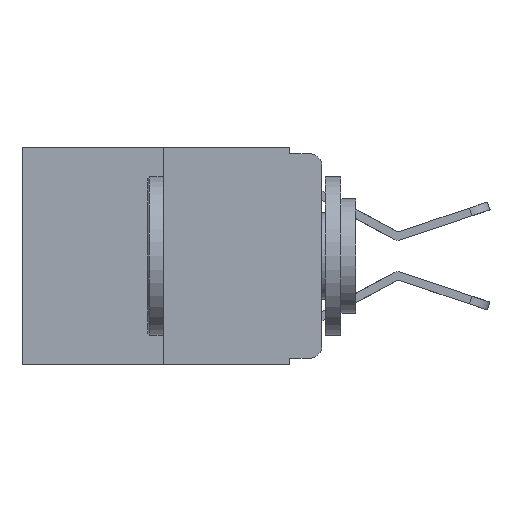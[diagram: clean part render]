
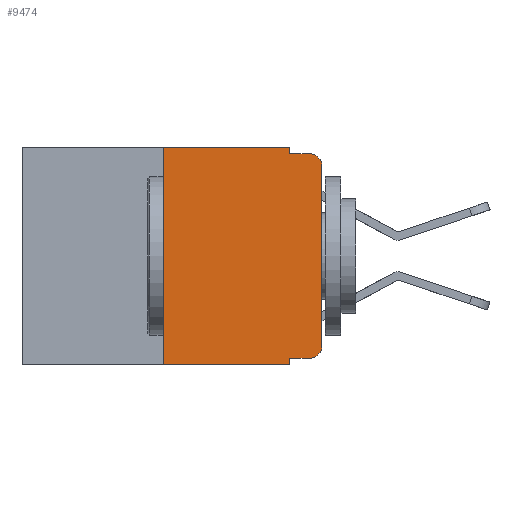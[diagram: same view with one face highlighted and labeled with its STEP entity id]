
A CAD part, left-side view. The second image highlights one B-rep face of the part: STEP entity #9474.
In plain terms, the highlighted planar face has unit normal (-1, 0, 0).
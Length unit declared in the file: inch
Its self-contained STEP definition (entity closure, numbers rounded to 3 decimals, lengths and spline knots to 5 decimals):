
#165 = DIRECTION ( 'NONE',  ( -1., 0., 0. ) ) ;
#377 = EDGE_CURVE ( 'NONE', #1621, #12043, #16840, .T. ) ;
#476 = CARTESIAN_POINT ( 'NONE',  ( 0., 0.051, -0.333 ) ) ;
#482 = CARTESIAN_POINT ( 'NONE',  ( 0., 0.051, -0.343 ) ) ;
#500 = VERTEX_POINT ( 'NONE', #15904 ) ;
#511 = EDGE_CURVE ( 'NONE', #15397, #2611, #18516, .T. ) ;
#589 = DIRECTION ( 'NONE',  ( 0., -1., 0. ) ) ;
#1621 = VERTEX_POINT ( 'NONE', #9645 ) ;
#1849 = PLANE ( 'NONE',  #20165 ) ;
#2248 = CIRCLE ( 'NONE', #12895, 0.02 ) ;
#2607 = CARTESIAN_POINT ( 'NONE',  ( 0., 0.473, -0.343 ) ) ;
#2611 = VERTEX_POINT ( 'NONE', #8493 ) ;
#2838 = ORIENTED_EDGE ( 'NONE', *, *, #20368, .T. ) ;
#3014 = VECTOR ( 'NONE', #19386, 39.37008 ) ;
#3291 = DIRECTION ( 'NONE',  ( 0., -1., 0. ) ) ;
#3378 = ORIENTED_EDGE ( 'NONE', *, *, #19338, .F. ) ;
#3545 = DIRECTION ( 'NONE',  ( 1., 0., 0. ) ) ;
#3826 = CARTESIAN_POINT ( 'NONE',  ( 0., 0.25, -0.343 ) ) ;
#3952 = VERTEX_POINT ( 'NONE', #3826 ) ;
#4013 = VECTOR ( 'NONE', #20763, 39.37008 ) ;
#4062 = VECTOR ( 'NONE', #3291, 39.37008 ) ;
#4450 = VECTOR ( 'NONE', #13975, 39.37008 ) ;
#4675 = EDGE_CURVE ( 'NONE', #3952, #16261, #12667, .T. ) ;
#5252 = ORIENTED_EDGE ( 'NONE', *, *, #16253, .F. ) ;
#5303 = DIRECTION ( 'NONE',  ( -1., 0., 0. ) ) ;
#5996 = ORIENTED_EDGE ( 'NONE', *, *, #18322, .F. ) ;
#6237 = ORIENTED_EDGE ( 'NONE', *, *, #511, .T. ) ;
#6366 = CARTESIAN_POINT ( 'NONE',  ( 0., 0., 0. ) ) ;
#6499 = ORIENTED_EDGE ( 'NONE', *, *, #377, .F. ) ;
#6713 = VECTOR ( 'NONE', #10400, 39.37008 ) ;
#6900 = CIRCLE ( 'NONE', #15809, 0.02 ) ;
#7520 = CARTESIAN_POINT ( 'NONE',  ( 0., 0.051, -0.333 ) ) ;
#7838 = FACE_OUTER_BOUND ( 'NONE', #12931, .T. ) ;
#8493 = CARTESIAN_POINT ( 'NONE',  ( 0., 0., -0.03 ) ) ;
#8799 = CARTESIAN_POINT ( 'NONE',  ( 0., 0.051, 0. ) ) ;
#8902 = CARTESIAN_POINT ( 'NONE',  ( 0., 0.051, -0.01 ) ) ;
#9474 = ADVANCED_FACE ( 'NONE', ( #7838 ), #1849, .F. ) ;
#9645 = CARTESIAN_POINT ( 'NONE',  ( 0., 0.25, 0. ) ) ;
#10112 = CARTESIAN_POINT ( 'NONE',  ( 0., 0.02, -0.03 ) ) ;
#10400 = DIRECTION ( 'NONE',  ( 0., 0., -1. ) ) ;
#10975 = VECTOR ( 'NONE', #589, 39.37008 ) ;
#10991 = LINE ( 'NONE', #18878, #15260 ) ;
#11568 = DIRECTION ( 'NONE',  ( 0., 0., 1. ) ) ;
#11703 = DIRECTION ( 'NONE',  ( 0., 0., -1. ) ) ;
#12043 = VERTEX_POINT ( 'NONE', #14399 ) ;
#12667 = LINE ( 'NONE', #2607, #4062 ) ;
#12895 = AXIS2_PLACEMENT_3D ( 'NONE', #14918, #5303, #16499 ) ;
#12931 = EDGE_LOOP ( 'NONE', ( #6237, #2838, #3378, #5996, #6499, #19642, #20609, #5252, #14808, #16291 ) ) ;
#13274 = CARTESIAN_POINT ( 'NONE',  ( 0., 0.473, 0. ) ) ;
#13975 = DIRECTION ( 'NONE',  ( 0., -1., 0. ) ) ;
#14120 = EDGE_CURVE ( 'NONE', #500, #15397, #2248, .T. ) ;
#14399 = CARTESIAN_POINT ( 'NONE',  ( 0., 0.051, 0. ) ) ;
#14584 = VERTEX_POINT ( 'NONE', #16076 ) ;
#14808 = ORIENTED_EDGE ( 'NONE', *, *, #15193, .T. ) ;
#14865 = VECTOR ( 'NONE', #11568, 39.37008 ) ;
#14873 = DIRECTION ( 'NONE',  ( 0., 0., -1. ) ) ;
#14918 = CARTESIAN_POINT ( 'NONE',  ( 0., 0.02, -0.313 ) ) ;
#15193 = EDGE_CURVE ( 'NONE', #18071, #500, #17744, .T. ) ;
#15260 = VECTOR ( 'NONE', #15777, 39.37008 ) ;
#15397 = VERTEX_POINT ( 'NONE', #20687 ) ;
#15777 = DIRECTION ( 'NONE',  ( 0., 0., -1. ) ) ;
#15809 = AXIS2_PLACEMENT_3D ( 'NONE', #10112, #165, #11703 ) ;
#15904 = CARTESIAN_POINT ( 'NONE',  ( 0., 0.02, -0.333 ) ) ;
#16076 = CARTESIAN_POINT ( 'NONE',  ( 0., 0.02, -0.01 ) ) ;
#16253 = EDGE_CURVE ( 'NONE', #18071, #16261, #19854, .T. ) ;
#16261 = VERTEX_POINT ( 'NONE', #482 ) ;
#16291 = ORIENTED_EDGE ( 'NONE', *, *, #14120, .T. ) ;
#16499 = DIRECTION ( 'NONE',  ( 0., 0., -1. ) ) ;
#16727 = CARTESIAN_POINT ( 'NONE',  ( 0., 0.473, 0. ) ) ;
#16840 = LINE ( 'NONE', #16727, #4013 ) ;
#17288 = EDGE_CURVE ( 'NONE', #3952, #1621, #20040, .T. ) ;
#17744 = LINE ( 'NONE', #7520, #4450 ) ;
#17855 = CARTESIAN_POINT ( 'NONE',  ( 0., 0.25, 0. ) ) ;
#18071 = VERTEX_POINT ( 'NONE', #476 ) ;
#18322 = EDGE_CURVE ( 'NONE', #12043, #18892, #10991, .T. ) ;
#18516 = LINE ( 'NONE', #6366, #14865 ) ;
#18878 = CARTESIAN_POINT ( 'NONE',  ( 0., 0.051, 0. ) ) ;
#18892 = VERTEX_POINT ( 'NONE', #20531 ) ;
#19338 = EDGE_CURVE ( 'NONE', #18892, #14584, #19349, .T. ) ;
#19349 = LINE ( 'NONE', #8902, #10975 ) ;
#19386 = DIRECTION ( 'NONE',  ( 0., 0., 1. ) ) ;
#19642 = ORIENTED_EDGE ( 'NONE', *, *, #17288, .F. ) ;
#19854 = LINE ( 'NONE', #8799, #6713 ) ;
#20040 = LINE ( 'NONE', #17855, #3014 ) ;
#20165 = AXIS2_PLACEMENT_3D ( 'NONE', #13274, #3545, #14873 ) ;
#20368 = EDGE_CURVE ( 'NONE', #2611, #14584, #6900, .T. ) ;
#20531 = CARTESIAN_POINT ( 'NONE',  ( 0., 0.051, -0.01 ) ) ;
#20609 = ORIENTED_EDGE ( 'NONE', *, *, #4675, .T. ) ;
#20687 = CARTESIAN_POINT ( 'NONE',  ( 0., 0., -0.313 ) ) ;
#20763 = DIRECTION ( 'NONE',  ( 0., -1., 0. ) ) ;
